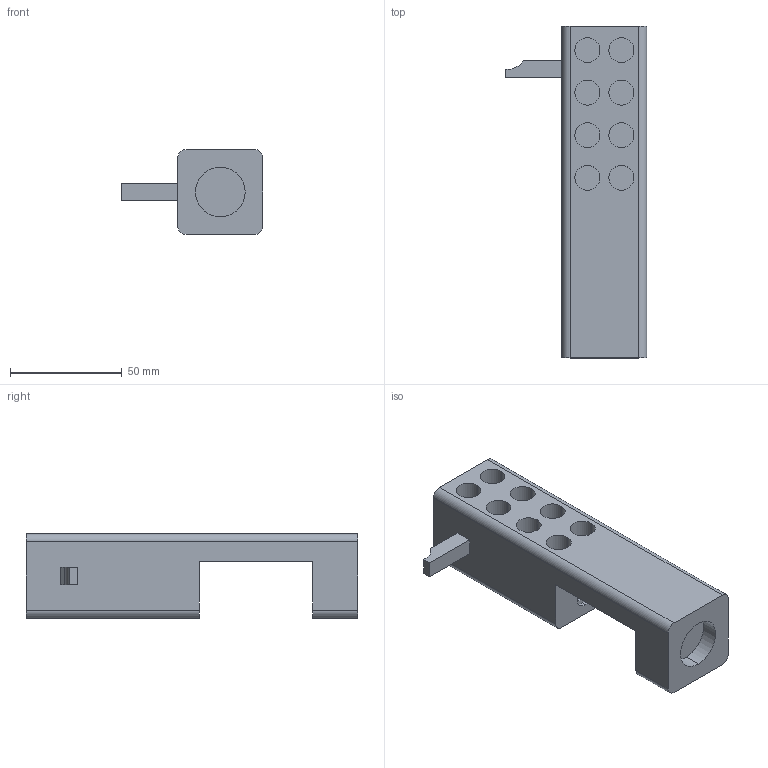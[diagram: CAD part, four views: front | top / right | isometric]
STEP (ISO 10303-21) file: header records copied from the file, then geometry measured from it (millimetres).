
FILE_DESCRIPTION (( 'STEP AP214' ), '1' );
FILE_NAME ('bolt.STEP', '2013-09-24T00:06:18', ( '' ), ( '' ), 'SwSTEP 2.0', 'SolidWorks 2013', '' );
FILE_SCHEMA (( 'AUTOMOTIVE_DESIGN' ));
Length unit declared in the file: inch
Products named in the file (1): bolt
Bounding box: 63.5 x 148.59 x 38.1 mm (x, y, z)
Volume: 144256.4 mm3; surface area: 32729.1 mm2
Topology: 1 solids, 1 shells, 70 faces, 167 edges, 110 vertices
Faces by surface type: plane 37, cylinder 33
Entity records: 2093 total; most frequent: DIRECTION 375, CARTESIAN_POINT 348, ORIENTED_EDGE 334, EDGE_CURVE 167, AXIS2_PLACEMENT_3D 137, VERTEX_POINT 110, LINE 101, VECTOR 101
